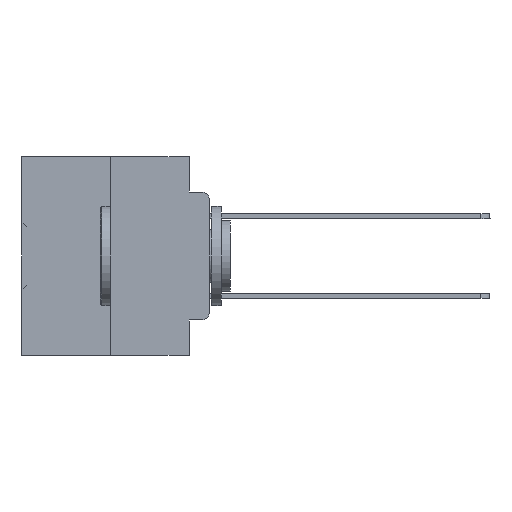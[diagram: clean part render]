
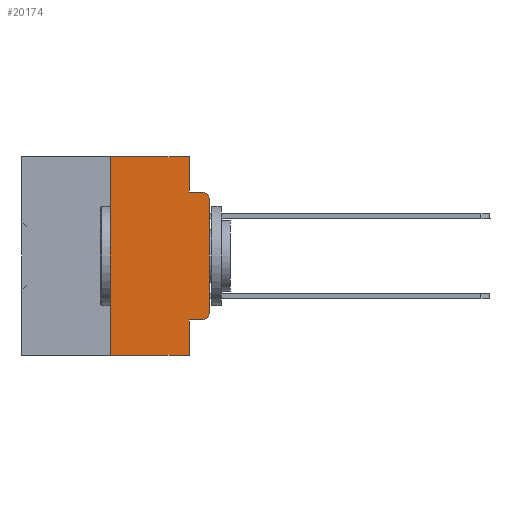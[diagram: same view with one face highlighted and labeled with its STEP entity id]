
A CAD part, left-side view. The second image highlights one B-rep face of the part: STEP entity #20174.
In plain terms, the highlighted planar face has unit normal (-1, 0, 0).
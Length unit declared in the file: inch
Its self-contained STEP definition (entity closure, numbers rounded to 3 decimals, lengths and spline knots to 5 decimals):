
#332 = VERTEX_POINT ( 'NONE', #5446 ) ;
#367 = VECTOR ( 'NONE', #3977, 39.37008 ) ;
#997 = CARTESIAN_POINT ( 'NONE',  ( 0., 0.02, -0.1085 ) ) ;
#1079 = VERTEX_POINT ( 'NONE', #3397 ) ;
#2606 = CARTESIAN_POINT ( 'NONE',  ( 0., 0.051, 0. ) ) ;
#2671 = CARTESIAN_POINT ( 'NONE',  ( 0., 0.051, 0. ) ) ;
#2855 = EDGE_LOOP ( 'NONE', ( #31371, #22843, #19835, #27111, #17170, #13896, #14530, #35642, #34603, #11011 ) ) ;
#3365 = CARTESIAN_POINT ( 'NONE',  ( 0., 0.051, -0.4115 ) ) ;
#3397 = CARTESIAN_POINT ( 'NONE',  ( 0., 0.02, -0.4115 ) ) ;
#3511 = VECTOR ( 'NONE', #5998, 39.37008 ) ;
#3726 = LINE ( 'NONE', #28736, #35934 ) ;
#3880 = DIRECTION ( 'NONE',  ( 1., 0., 0. ) ) ;
#3897 = CARTESIAN_POINT ( 'NONE',  ( 0., 0.051, -0.5 ) ) ;
#3967 = EDGE_CURVE ( 'NONE', #38335, #1079, #26751, .T. ) ;
#3977 = DIRECTION ( 'NONE',  ( 0., 0., 1. ) ) ;
#5398 = VERTEX_POINT ( 'NONE', #3897 ) ;
#5446 = CARTESIAN_POINT ( 'NONE',  ( 0., 0.25, -0.5 ) ) ;
#5949 = AXIS2_PLACEMENT_3D ( 'NONE', #997, #10956, #25781 ) ;
#5998 = DIRECTION ( 'NONE',  ( 0., -1., 0. ) ) ;
#6718 = EDGE_CURVE ( 'NONE', #36226, #23938, #3726, .T. ) ;
#7834 = EDGE_CURVE ( 'NONE', #10143, #25323, #15031, .T. ) ;
#9413 = VECTOR ( 'NONE', #23377, 39.37008 ) ;
#9998 = LINE ( 'NONE', #2606, #13852 ) ;
#10143 = VERTEX_POINT ( 'NONE', #24529 ) ;
#10403 = EDGE_CURVE ( 'NONE', #38335, #5398, #10852, .T. ) ;
#10505 = LINE ( 'NONE', #37795, #16181 ) ;
#10852 = LINE ( 'NONE', #36029, #9413 ) ;
#10956 = DIRECTION ( 'NONE',  ( -1., 0., 0. ) ) ;
#11011 = ORIENTED_EDGE ( 'NONE', *, *, #19694, .T. ) ;
#11220 = DIRECTION ( 'NONE',  ( -1., 0., 0. ) ) ;
#12207 = VERTEX_POINT ( 'NONE', #13474 ) ;
#13371 = DIRECTION ( 'NONE',  ( 0., -1., 0. ) ) ;
#13474 = CARTESIAN_POINT ( 'NONE',  ( 0., 0., -0.3915 ) ) ;
#13852 = VECTOR ( 'NONE', #20905, 39.37008 ) ;
#13896 = ORIENTED_EDGE ( 'NONE', *, *, #20830, .F. ) ;
#14018 = CARTESIAN_POINT ( 'NONE',  ( 0., 0.02, -0.3915 ) ) ;
#14530 = ORIENTED_EDGE ( 'NONE', *, *, #28091, .T. ) ;
#14593 = VECTOR ( 'NONE', #17560, 39.37008 ) ;
#15031 = LINE ( 'NONE', #35663, #14593 ) ;
#15128 = CARTESIAN_POINT ( 'NONE',  ( 0., 0.473, -0.5 ) ) ;
#16181 = VECTOR ( 'NONE', #19815, 39.37008 ) ;
#16238 = DIRECTION ( 'NONE',  ( 0., -1., 0. ) ) ;
#17170 = ORIENTED_EDGE ( 'NONE', *, *, #7834, .F. ) ;
#17560 = DIRECTION ( 'NONE',  ( 0., -1., 0. ) ) ;
#17829 = CARTESIAN_POINT ( 'NONE',  ( 0., 0.02, -0.0885 ) ) ;
#18761 = AXIS2_PLACEMENT_3D ( 'NONE', #14018, #11220, #32538 ) ;
#19694 = EDGE_CURVE ( 'NONE', #1079, #12207, #36002, .T. ) ;
#19815 = DIRECTION ( 'NONE',  ( 0., 0., 1. ) ) ;
#19835 = ORIENTED_EDGE ( 'NONE', *, *, #6718, .F. ) ;
#20174 = ADVANCED_FACE ( 'NONE', ( #32704 ), #30904, .F. ) ;
#20398 = CIRCLE ( 'NONE', #5949, 0.02 ) ;
#20830 = EDGE_CURVE ( 'NONE', #332, #10143, #22200, .T. ) ;
#20905 = DIRECTION ( 'NONE',  ( 0., 0., -1. ) ) ;
#21973 = VECTOR ( 'NONE', #13371, 39.37008 ) ;
#22200 = LINE ( 'NONE', #25013, #367 ) ;
#22843 = ORIENTED_EDGE ( 'NONE', *, *, #25066, .T. ) ;
#23122 = EDGE_CURVE ( 'NONE', #12207, #32745, #10505, .T. ) ;
#23377 = DIRECTION ( 'NONE',  ( 0., 0., -1. ) ) ;
#23938 = VERTEX_POINT ( 'NONE', #17829 ) ;
#24529 = CARTESIAN_POINT ( 'NONE',  ( 0., 0.25, 0. ) ) ;
#25013 = CARTESIAN_POINT ( 'NONE',  ( 0., 0.25, 0. ) ) ;
#25042 = CARTESIAN_POINT ( 'NONE',  ( 0., 0.473, 0. ) ) ;
#25066 = EDGE_CURVE ( 'NONE', #32745, #23938, #20398, .T. ) ;
#25185 = DIRECTION ( 'NONE',  ( 0., 0., -1. ) ) ;
#25323 = VERTEX_POINT ( 'NONE', #2671 ) ;
#25781 = DIRECTION ( 'NONE',  ( 0., 0., -1. ) ) ;
#26294 = LINE ( 'NONE', #15128, #3511 ) ;
#26751 = LINE ( 'NONE', #37154, #21973 ) ;
#27111 = ORIENTED_EDGE ( 'NONE', *, *, #36456, .F. ) ;
#28091 = EDGE_CURVE ( 'NONE', #332, #5398, #26294, .T. ) ;
#28167 = AXIS2_PLACEMENT_3D ( 'NONE', #25042, #3880, #25185 ) ;
#28736 = CARTESIAN_POINT ( 'NONE',  ( 0., 0.051, -0.0885 ) ) ;
#29302 = CARTESIAN_POINT ( 'NONE',  ( 0., 0., -0.1085 ) ) ;
#30904 = PLANE ( 'NONE',  #28167 ) ;
#31371 = ORIENTED_EDGE ( 'NONE', *, *, #23122, .T. ) ;
#32538 = DIRECTION ( 'NONE',  ( 0., 0., -1. ) ) ;
#32704 = FACE_OUTER_BOUND ( 'NONE', #2855, .T. ) ;
#32745 = VERTEX_POINT ( 'NONE', #29302 ) ;
#34603 = ORIENTED_EDGE ( 'NONE', *, *, #3967, .T. ) ;
#34648 = CARTESIAN_POINT ( 'NONE',  ( 0., 0.051, -0.0885 ) ) ;
#35642 = ORIENTED_EDGE ( 'NONE', *, *, #10403, .F. ) ;
#35663 = CARTESIAN_POINT ( 'NONE',  ( 0., 0.473, 0. ) ) ;
#35934 = VECTOR ( 'NONE', #16238, 39.37008 ) ;
#36002 = CIRCLE ( 'NONE', #18761, 0.02 ) ;
#36029 = CARTESIAN_POINT ( 'NONE',  ( 0., 0.051, 0. ) ) ;
#36226 = VERTEX_POINT ( 'NONE', #34648 ) ;
#36456 = EDGE_CURVE ( 'NONE', #25323, #36226, #9998, .T. ) ;
#37154 = CARTESIAN_POINT ( 'NONE',  ( 0., 0.051, -0.4115 ) ) ;
#37795 = CARTESIAN_POINT ( 'NONE',  ( 0., 0., 0. ) ) ;
#38335 = VERTEX_POINT ( 'NONE', #3365 ) ;
